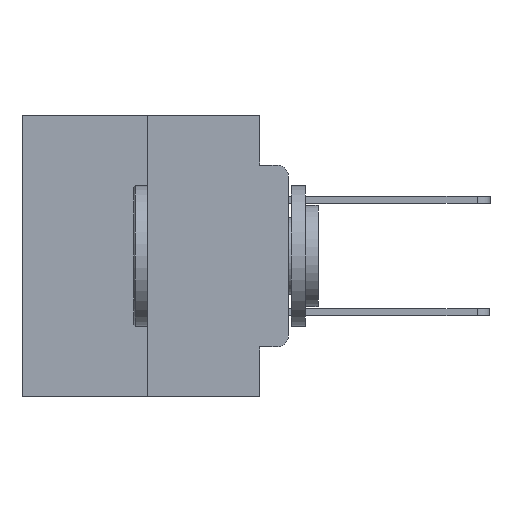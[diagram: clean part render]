
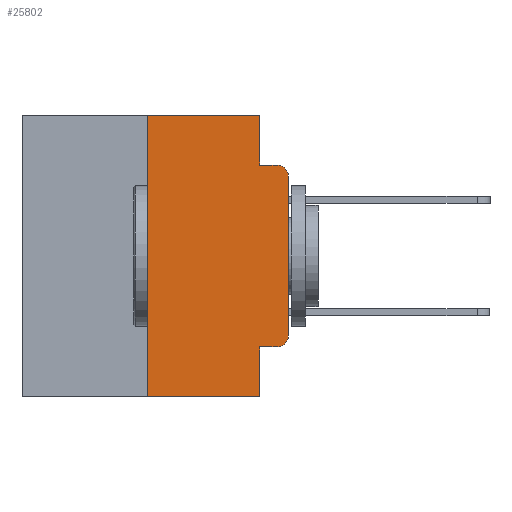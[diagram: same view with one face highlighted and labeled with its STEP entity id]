
A CAD part, left-side view. The second image highlights one B-rep face of the part: STEP entity #25802.
In plain terms, the highlighted planar face has unit normal (-1, 0, 0).
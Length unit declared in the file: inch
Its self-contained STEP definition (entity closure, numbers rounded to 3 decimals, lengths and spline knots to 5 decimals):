
#337 = DIRECTION ( 'NONE',  ( 1., 0., 0. ) ) ;
#397 = AXIS2_PLACEMENT_3D ( 'NONE', #11840, #26735, #13968 ) ;
#401 = LINE ( 'NONE', #13793, #5762 ) ;
#476 = VERTEX_POINT ( 'NONE', #20106 ) ;
#605 = EDGE_CURVE ( 'NONE', #10428, #22650, #20597, .T. ) ;
#868 = ORIENTED_EDGE ( 'NONE', *, *, #24739, .F. ) ;
#967 = EDGE_CURVE ( 'NONE', #476, #3657, #7501, .T. ) ;
#1818 = AXIS2_PLACEMENT_3D ( 'NONE', #16528, #3611, #18651 ) ;
#1864 = VERTEX_POINT ( 'NONE', #8117 ) ;
#2949 = DIRECTION ( 'NONE',  ( 0., 0., 1. ) ) ;
#3319 = LINE ( 'NONE', #20005, #14152 ) ;
#3563 = LINE ( 'NONE', #22857, #25747 ) ;
#3611 = DIRECTION ( 'NONE',  ( -1., 0., 0. ) ) ;
#3657 = VERTEX_POINT ( 'NONE', #18529 ) ;
#4080 = EDGE_CURVE ( 'NONE', #9977, #3657, #12681, .T. ) ;
#4215 = CARTESIAN_POINT ( 'NONE',  ( 0., 0., -0.3915 ) ) ;
#5050 = DIRECTION ( 'NONE',  ( 0., 0., -1. ) ) ;
#5762 = VECTOR ( 'NONE', #2949, 39.37008 ) ;
#6677 = LINE ( 'NONE', #22620, #23026 ) ;
#7180 = CARTESIAN_POINT ( 'NONE',  ( 0., 0.051, -0.5 ) ) ;
#7271 = ORIENTED_EDGE ( 'NONE', *, *, #21493, .F. ) ;
#7501 = LINE ( 'NONE', #10770, #17507 ) ;
#7649 = DIRECTION ( 'NONE',  ( 0., -1., 0. ) ) ;
#8117 = CARTESIAN_POINT ( 'NONE',  ( 0., 0.051, -0.4115 ) ) ;
#8791 = CARTESIAN_POINT ( 'NONE',  ( 0., 0.25, 0. ) ) ;
#9275 = VECTOR ( 'NONE', #12004, 39.37008 ) ;
#9403 = EDGE_CURVE ( 'NONE', #17430, #25001, #21503, .T. ) ;
#9600 = CARTESIAN_POINT ( 'NONE',  ( 0., 0.473, -0.5 ) ) ;
#9977 = VERTEX_POINT ( 'NONE', #16405 ) ;
#10061 = DIRECTION ( 'NONE',  ( 0., -1., 0. ) ) ;
#10144 = VECTOR ( 'NONE', #7649, 39.37008 ) ;
#10428 = VERTEX_POINT ( 'NONE', #15826 ) ;
#10770 = CARTESIAN_POINT ( 'NONE',  ( 0., 0.051, -0.0885 ) ) ;
#11287 = DIRECTION ( 'NONE',  ( 0., 0., 1. ) ) ;
#11840 = CARTESIAN_POINT ( 'NONE',  ( 0., 0.02, -0.1085 ) ) ;
#12004 = DIRECTION ( 'NONE',  ( 0., -1., 0. ) ) ;
#12625 = ORIENTED_EDGE ( 'NONE', *, *, #20950, .F. ) ;
#12681 = CIRCLE ( 'NONE', #397, 0.02 ) ;
#13228 = LINE ( 'NONE', #21896, #22545 ) ;
#13678 = VERTEX_POINT ( 'NONE', #20565 ) ;
#13793 = CARTESIAN_POINT ( 'NONE',  ( 0., 0., 0. ) ) ;
#13968 = DIRECTION ( 'NONE',  ( 0., 0., -1. ) ) ;
#14152 = VECTOR ( 'NONE', #5050, 39.37008 ) ;
#14192 = FACE_OUTER_BOUND ( 'NONE', #17915, .T. ) ;
#15097 = ORIENTED_EDGE ( 'NONE', *, *, #16503, .T. ) ;
#15562 = CARTESIAN_POINT ( 'NONE',  ( 0., 0.473, 0. ) ) ;
#15595 = VERTEX_POINT ( 'NONE', #4215 ) ;
#15652 = DIRECTION ( 'NONE',  ( 0., 0., -1. ) ) ;
#15826 = CARTESIAN_POINT ( 'NONE',  ( 0., 0.25, -0.5 ) ) ;
#16405 = CARTESIAN_POINT ( 'NONE',  ( 0., 0., -0.1085 ) ) ;
#16503 = EDGE_CURVE ( 'NONE', #15595, #9977, #401, .T. ) ;
#16528 = CARTESIAN_POINT ( 'NONE',  ( 0., 0.02, -0.3915 ) ) ;
#16580 = ORIENTED_EDGE ( 'NONE', *, *, #9403, .F. ) ;
#16762 = CIRCLE ( 'NONE', #1818, 0.02 ) ;
#17211 = EDGE_CURVE ( 'NONE', #13678, #15595, #16762, .T. ) ;
#17430 = VERTEX_POINT ( 'NONE', #8791 ) ;
#17507 = VECTOR ( 'NONE', #22003, 39.37008 ) ;
#17915 = EDGE_LOOP ( 'NONE', ( #15097, #27791, #25583, #868, #16580, #12625, #24631, #7271, #20607, #20683 ) ) ;
#18279 = CARTESIAN_POINT ( 'NONE',  ( 0., 0.473, 0. ) ) ;
#18529 = CARTESIAN_POINT ( 'NONE',  ( 0., 0.02, -0.0885 ) ) ;
#18613 = EDGE_CURVE ( 'NONE', #1864, #13678, #3563, .T. ) ;
#18651 = DIRECTION ( 'NONE',  ( 0., 0., -1. ) ) ;
#19224 = CARTESIAN_POINT ( 'NONE',  ( 0., 0.051, 0. ) ) ;
#20005 = CARTESIAN_POINT ( 'NONE',  ( 0., 0.051, 0. ) ) ;
#20106 = CARTESIAN_POINT ( 'NONE',  ( 0., 0.051, -0.0885 ) ) ;
#20565 = CARTESIAN_POINT ( 'NONE',  ( 0., 0.02, -0.4115 ) ) ;
#20597 = LINE ( 'NONE', #9600, #9275 ) ;
#20607 = ORIENTED_EDGE ( 'NONE', *, *, #18613, .T. ) ;
#20683 = ORIENTED_EDGE ( 'NONE', *, *, #17211, .T. ) ;
#20950 = EDGE_CURVE ( 'NONE', #10428, #17430, #13228, .T. ) ;
#21493 = EDGE_CURVE ( 'NONE', #1864, #22650, #3319, .T. ) ;
#21503 = LINE ( 'NONE', #18279, #10144 ) ;
#21896 = CARTESIAN_POINT ( 'NONE',  ( 0., 0.25, 0. ) ) ;
#21997 = PLANE ( 'NONE',  #22187 ) ;
#22003 = DIRECTION ( 'NONE',  ( 0., -1., 0. ) ) ;
#22187 = AXIS2_PLACEMENT_3D ( 'NONE', #15562, #337, #15652 ) ;
#22545 = VECTOR ( 'NONE', #11287, 39.37008 ) ;
#22620 = CARTESIAN_POINT ( 'NONE',  ( 0., 0.051, 0. ) ) ;
#22650 = VERTEX_POINT ( 'NONE', #7180 ) ;
#22857 = CARTESIAN_POINT ( 'NONE',  ( 0., 0.051, -0.4115 ) ) ;
#23026 = VECTOR ( 'NONE', #24855, 39.37008 ) ;
#24631 = ORIENTED_EDGE ( 'NONE', *, *, #605, .T. ) ;
#24739 = EDGE_CURVE ( 'NONE', #25001, #476, #6677, .T. ) ;
#24855 = DIRECTION ( 'NONE',  ( 0., 0., -1. ) ) ;
#25001 = VERTEX_POINT ( 'NONE', #19224 ) ;
#25583 = ORIENTED_EDGE ( 'NONE', *, *, #967, .F. ) ;
#25747 = VECTOR ( 'NONE', #10061, 39.37008 ) ;
#25802 = ADVANCED_FACE ( 'NONE', ( #14192 ), #21997, .F. ) ;
#26735 = DIRECTION ( 'NONE',  ( -1., 0., 0. ) ) ;
#27791 = ORIENTED_EDGE ( 'NONE', *, *, #4080, .T. ) ;
